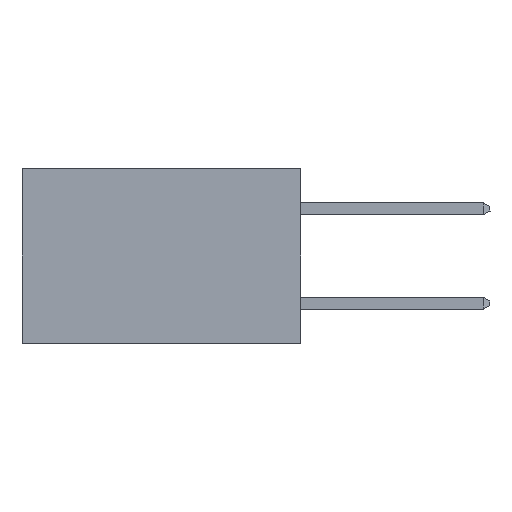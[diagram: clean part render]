
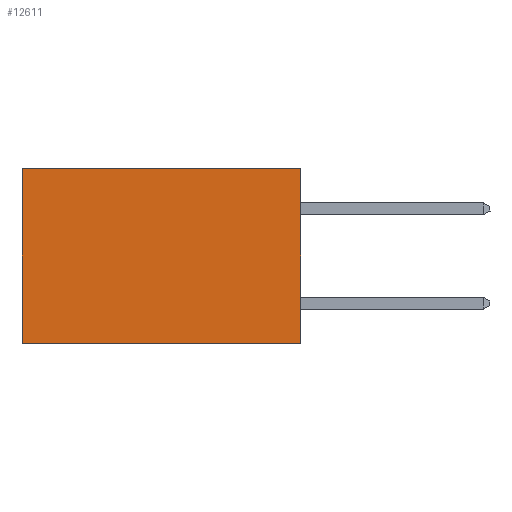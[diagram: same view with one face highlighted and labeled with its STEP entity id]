
A CAD part, left-side view. The second image highlights one B-rep face of the part: STEP entity #12611.
In plain terms, the highlighted planar face has unit normal (-1, 0, 0).
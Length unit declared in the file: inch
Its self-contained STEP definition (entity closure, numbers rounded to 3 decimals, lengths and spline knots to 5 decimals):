
#1525 = CARTESIAN_POINT ( 'NONE',  ( 0.277, 0.59, -0.37 ) ) ;
#3150 = DIRECTION ( 'NONE',  ( 0., 0., -1. ) ) ;
#3443 = VERTEX_POINT ( 'NONE', #5052 ) ;
#5052 = CARTESIAN_POINT ( 'NONE',  ( 0.277, 0., -0.37 ) ) ;
#5245 = VECTOR ( 'NONE', #7651, 39.37008 ) ;
#5367 = DIRECTION ( 'NONE',  ( 0., 1., 0. ) ) ;
#5378 = VECTOR ( 'NONE', #5367, 39.37008 ) ;
#5868 = AXIS2_PLACEMENT_3D ( 'NONE', #8008, #10481, #3150 ) ;
#5966 = ORIENTED_EDGE ( 'NONE', *, *, #12724, .T. ) ;
#6027 = LINE ( 'NONE', #6420, #5245 ) ;
#6420 = CARTESIAN_POINT ( 'NONE',  ( 0.277, 0., 0. ) ) ;
#7651 = DIRECTION ( 'NONE',  ( 0., 1., 0. ) ) ;
#7896 = VERTEX_POINT ( 'NONE', #10329 ) ;
#7907 = ORIENTED_EDGE ( 'NONE', *, *, #15150, .F. ) ;
#8008 = CARTESIAN_POINT ( 'NONE',  ( 0.277, 0., -0.37 ) ) ;
#8651 = LINE ( 'NONE', #15046, #5378 ) ;
#9028 = DIRECTION ( 'NONE',  ( 0., 0., -1. ) ) ;
#9276 = PLANE ( 'NONE',  #5868 ) ;
#10321 = ORIENTED_EDGE ( 'NONE', *, *, #11895, .F. ) ;
#10329 = CARTESIAN_POINT ( 'NONE',  ( 0.277, 0., 0. ) ) ;
#10481 = DIRECTION ( 'NONE',  ( 1., 0., 0. ) ) ;
#10616 = VECTOR ( 'NONE', #9028, 39.37008 ) ;
#11003 = ORIENTED_EDGE ( 'NONE', *, *, #11840, .T. ) ;
#11165 = VERTEX_POINT ( 'NONE', #1525 ) ;
#11418 = VECTOR ( 'NONE', #15456, 39.37008 ) ;
#11840 = EDGE_CURVE ( 'NONE', #7896, #12862, #6027, .T. ) ;
#11895 = EDGE_CURVE ( 'NONE', #7896, #3443, #13812, .T. ) ;
#12346 = EDGE_LOOP ( 'NONE', ( #5966, #7907, #10321, #11003 ) ) ;
#12611 = ADVANCED_FACE ( 'NONE', ( #13309 ), #9276, .F. ) ;
#12724 = EDGE_CURVE ( 'NONE', #12862, #11165, #14598, .T. ) ;
#12862 = VERTEX_POINT ( 'NONE', #14488 ) ;
#13309 = FACE_OUTER_BOUND ( 'NONE', #12346, .T. ) ;
#13809 = CARTESIAN_POINT ( 'NONE',  ( 0.277, 0., -0.37 ) ) ;
#13812 = LINE ( 'NONE', #13809, #10616 ) ;
#14488 = CARTESIAN_POINT ( 'NONE',  ( 0.277, 0.59, 0. ) ) ;
#14598 = LINE ( 'NONE', #15408, #11418 ) ;
#15046 = CARTESIAN_POINT ( 'NONE',  ( 0.277, 0., -0.37 ) ) ;
#15150 = EDGE_CURVE ( 'NONE', #3443, #11165, #8651, .T. ) ;
#15408 = CARTESIAN_POINT ( 'NONE',  ( 0.277, 0.59, -0.37 ) ) ;
#15456 = DIRECTION ( 'NONE',  ( 0., 0., -1. ) ) ;
